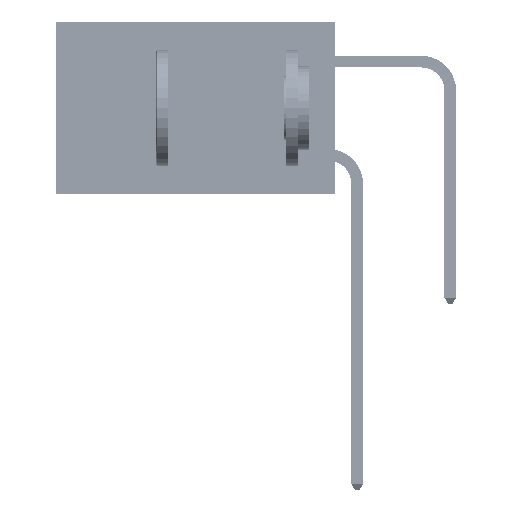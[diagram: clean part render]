
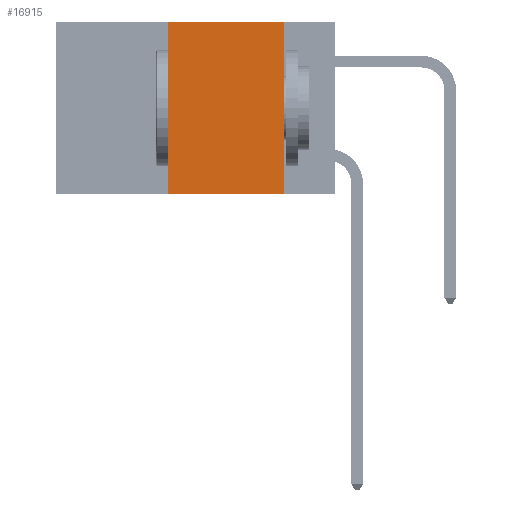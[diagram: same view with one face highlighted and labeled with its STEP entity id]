
A CAD part, left-side view. The second image highlights one B-rep face of the part: STEP entity #16915.
In plain terms, the highlighted planar face has unit normal (-1, 0, 0).
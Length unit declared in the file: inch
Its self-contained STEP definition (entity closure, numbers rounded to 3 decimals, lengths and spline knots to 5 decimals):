
#1510 = ORIENTED_EDGE ( 'NONE', *, *, #38007, .F. ) ;
#3754 = AXIS2_PLACEMENT_3D ( 'NONE', #15888, #12093, #27323 ) ;
#3869 = CARTESIAN_POINT ( 'NONE',  ( 0., 0.11, 0. ) ) ;
#4064 = VECTOR ( 'NONE', #9576, 39.37008 ) ;
#4138 = EDGE_CURVE ( 'NONE', #7404, #25719, #24329, .T. ) ;
#4543 = CARTESIAN_POINT ( 'NONE',  ( 0., 0.11, -0.37 ) ) ;
#5138 = DIRECTION ( 'NONE',  ( 0., 0., 1. ) ) ;
#5428 = ORIENTED_EDGE ( 'NONE', *, *, #4138, .F. ) ;
#6317 = EDGE_CURVE ( 'NONE', #9819, #7404, #44915, .T. ) ;
#7404 = VERTEX_POINT ( 'NONE', #36493 ) ;
#9576 = DIRECTION ( 'NONE',  ( 0., -1., 0. ) ) ;
#9812 = FACE_OUTER_BOUND ( 'NONE', #39000, .T. ) ;
#9819 = VERTEX_POINT ( 'NONE', #11041 ) ;
#11041 = CARTESIAN_POINT ( 'NONE',  ( 0., 0.36, 0. ) ) ;
#12093 = DIRECTION ( 'NONE',  ( 1., 0., 0. ) ) ;
#12731 = CARTESIAN_POINT ( 'NONE',  ( 0., 0.6, 0. ) ) ;
#13434 = ORIENTED_EDGE ( 'NONE', *, *, #6317, .F. ) ;
#15888 = CARTESIAN_POINT ( 'NONE',  ( 0., 0.6, 0. ) ) ;
#16915 = ADVANCED_FACE ( 'NONE', ( #9812 ), #27487, .F. ) ;
#17696 = LINE ( 'NONE', #43349, #18279 ) ;
#18279 = VECTOR ( 'NONE', #5138, 39.37008 ) ;
#19241 = DIRECTION ( 'NONE',  ( 0., 0., -1. ) ) ;
#21235 = VECTOR ( 'NONE', #45490, 39.37008 ) ;
#22306 = CARTESIAN_POINT ( 'NONE',  ( 0., 0.6, -0.37 ) ) ;
#24329 = LINE ( 'NONE', #3869, #42115 ) ;
#25719 = VERTEX_POINT ( 'NONE', #4543 ) ;
#27323 = DIRECTION ( 'NONE',  ( 0., 0., -1. ) ) ;
#27487 = PLANE ( 'NONE',  #3754 ) ;
#27698 = ORIENTED_EDGE ( 'NONE', *, *, #38302, .T. ) ;
#30137 = LINE ( 'NONE', #22306, #21235 ) ;
#36493 = CARTESIAN_POINT ( 'NONE',  ( 0., 0.11, 0. ) ) ;
#37724 = CARTESIAN_POINT ( 'NONE',  ( 0., 0.36, -0.37 ) ) ;
#38007 = EDGE_CURVE ( 'NONE', #38359, #9819, #17696, .T. ) ;
#38302 = EDGE_CURVE ( 'NONE', #38359, #25719, #30137, .T. ) ;
#38359 = VERTEX_POINT ( 'NONE', #37724 ) ;
#39000 = EDGE_LOOP ( 'NONE', ( #5428, #13434, #1510, #27698 ) ) ;
#42115 = VECTOR ( 'NONE', #19241, 39.37008 ) ;
#43349 = CARTESIAN_POINT ( 'NONE',  ( 0., 0.36, 0. ) ) ;
#44915 = LINE ( 'NONE', #12731, #4064 ) ;
#45490 = DIRECTION ( 'NONE',  ( 0., -1., 0. ) ) ;
